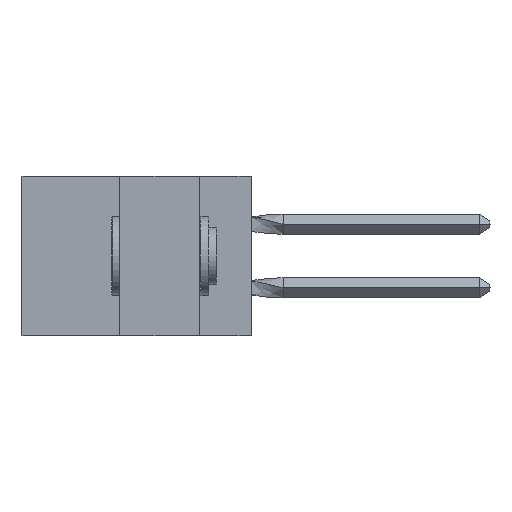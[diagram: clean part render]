
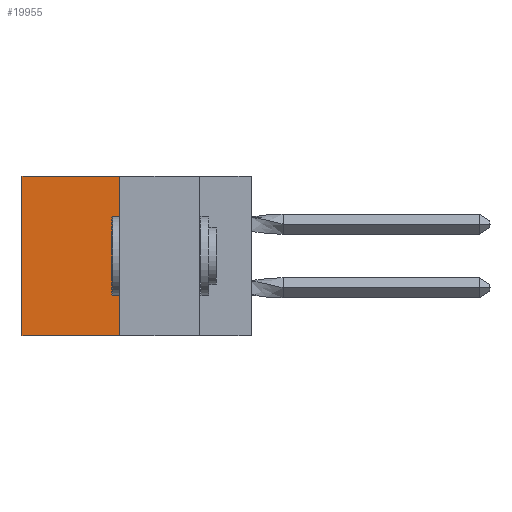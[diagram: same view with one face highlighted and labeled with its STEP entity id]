
A CAD part, left-side view. The second image highlights one B-rep face of the part: STEP entity #19955.
In plain terms, the highlighted planar face has unit normal (-1, 0, 0).
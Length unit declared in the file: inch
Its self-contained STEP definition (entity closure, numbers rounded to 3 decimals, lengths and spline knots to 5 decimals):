
#974 = VERTEX_POINT ( 'NONE', #12690 ) ;
#1828 = LINE ( 'NONE', #23577, #16554 ) ;
#2999 = CARTESIAN_POINT ( 'NONE',  ( 0.305, 0.413, -0.5 ) ) ;
#3829 = ORIENTED_EDGE ( 'NONE', *, *, #17005, .F. ) ;
#5207 = DIRECTION ( 'NONE',  ( 1., 0., 0. ) ) ;
#5775 = CARTESIAN_POINT ( 'NONE',  ( 0.305, 0.413, -0.5 ) ) ;
#7864 = EDGE_CURVE ( 'NONE', #974, #25366, #21432, .T. ) ;
#9407 = FACE_OUTER_BOUND ( 'NONE', #18180, .T. ) ;
#9473 = ORIENTED_EDGE ( 'NONE', *, *, #25836, .F. ) ;
#10078 = DIRECTION ( 'NONE',  ( 0., 1., 0. ) ) ;
#11235 = LINE ( 'NONE', #17401, #24217 ) ;
#11334 = LINE ( 'NONE', #5775, #27016 ) ;
#11348 = EDGE_CURVE ( 'NONE', #25366, #12770, #11235, .T. ) ;
#12690 = CARTESIAN_POINT ( 'NONE',  ( 0.305, 0.413, 0. ) ) ;
#12770 = VERTEX_POINT ( 'NONE', #20230 ) ;
#12917 = DIRECTION ( 'NONE',  ( 0., 1., 0. ) ) ;
#12934 = VERTEX_POINT ( 'NONE', #2999 ) ;
#13497 = DIRECTION ( 'NONE',  ( 0., 0., -1. ) ) ;
#16554 = VECTOR ( 'NONE', #21062, 39.37008 ) ;
#17005 = EDGE_CURVE ( 'NONE', #974, #12934, #1828, .T. ) ;
#17401 = CARTESIAN_POINT ( 'NONE',  ( 0.305, 0.72, -0.5 ) ) ;
#17532 = AXIS2_PLACEMENT_3D ( 'NONE', #17927, #5207, #18117 ) ;
#17927 = CARTESIAN_POINT ( 'NONE',  ( 0.305, 0.413, -0.5 ) ) ;
#18117 = DIRECTION ( 'NONE',  ( 0., 0., -1. ) ) ;
#18180 = EDGE_LOOP ( 'NONE', ( #20660, #9473, #3829, #19417 ) ) ;
#18438 = VECTOR ( 'NONE', #12917, 39.37008 ) ;
#18478 = CARTESIAN_POINT ( 'NONE',  ( 0.305, 0.72, 0. ) ) ;
#19417 = ORIENTED_EDGE ( 'NONE', *, *, #7864, .T. ) ;
#19955 = ADVANCED_FACE ( 'NONE', ( #9407 ), #26698, .F. ) ;
#20230 = CARTESIAN_POINT ( 'NONE',  ( 0.305, 0.72, -0.5 ) ) ;
#20660 = ORIENTED_EDGE ( 'NONE', *, *, #11348, .T. ) ;
#21062 = DIRECTION ( 'NONE',  ( 0., 0., -1. ) ) ;
#21432 = LINE ( 'NONE', #25912, #18438 ) ;
#23577 = CARTESIAN_POINT ( 'NONE',  ( 0.305, 0.413, -0.5 ) ) ;
#24217 = VECTOR ( 'NONE', #13497, 39.37008 ) ;
#25366 = VERTEX_POINT ( 'NONE', #18478 ) ;
#25836 = EDGE_CURVE ( 'NONE', #12934, #12770, #11334, .T. ) ;
#25912 = CARTESIAN_POINT ( 'NONE',  ( 0.305, 0.413, 0. ) ) ;
#26698 = PLANE ( 'NONE',  #17532 ) ;
#27016 = VECTOR ( 'NONE', #10078, 39.37008 ) ;
